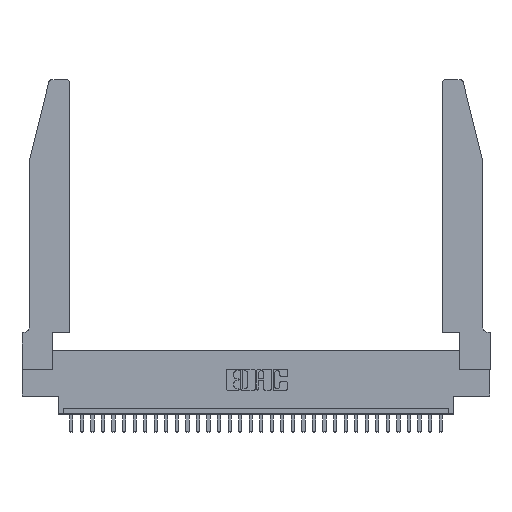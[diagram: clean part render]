
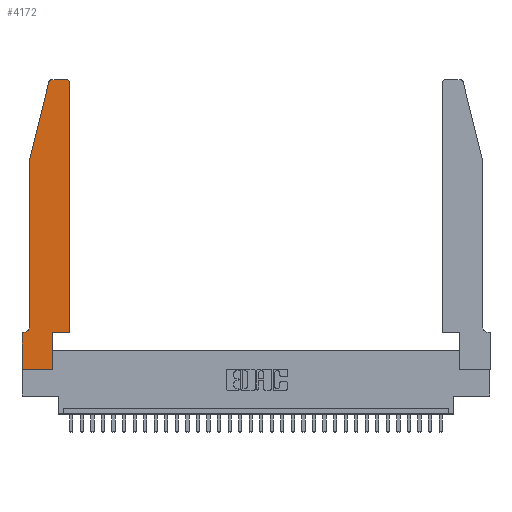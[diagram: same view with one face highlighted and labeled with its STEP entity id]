
A CAD part, top view. The second image highlights one B-rep face of the part: STEP entity #4172.
In plain terms, the highlighted planar face has unit normal (0, 0, 1).
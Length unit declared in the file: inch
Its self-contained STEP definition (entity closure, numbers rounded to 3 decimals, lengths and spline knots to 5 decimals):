
#710 = ORIENTED_EDGE ( 'NONE', *, *, #9412, .T. ) ;
#775 = AXIS2_PLACEMENT_3D ( 'NONE', #27414, #29863, #1965 ) ;
#939 = VECTOR ( 'NONE', #19447, 39.37008 ) ;
#1406 = CARTESIAN_POINT ( 'NONE',  ( 0.0755, 0.35, 0.37 ) ) ;
#1435 = ORIENTED_EDGE ( 'NONE', *, *, #9471, .T. ) ;
#1589 = DIRECTION ( 'NONE',  ( -0.239, -0.971, 0. ) ) ;
#1730 = VERTEX_POINT ( 'NONE', #30564 ) ;
#1965 = DIRECTION ( 'NONE',  ( -1., 0., 0. ) ) ;
#2129 = VERTEX_POINT ( 'NONE', #17123 ) ;
#2158 = CARTESIAN_POINT ( 'NONE',  ( 0.4505, 0.35, 0.37 ) ) ;
#2276 = EDGE_LOOP ( 'NONE', ( #29043, #710, #28399, #22956, #30868, #19934, #21627, #17759, #14311, #11859, #1435, #21307 ) ) ;
#2310 = CARTESIAN_POINT ( 'NONE',  ( 0., 0., 0.37 ) ) ;
#2598 = DIRECTION ( 'NONE',  ( 0., -1., 0. ) ) ;
#2951 = CARTESIAN_POINT ( 'NONE',  ( 0., 0., 0.37 ) ) ;
#3043 = DIRECTION ( 'NONE',  ( 0., -1., 0. ) ) ;
#3493 = VERTEX_POINT ( 'NONE', #13607 ) ;
#4172 = ADVANCED_FACE ( 'NONE', ( #28585 ), #24012, .T. ) ;
#4208 = DIRECTION ( 'NONE',  ( 0., 0., 1. ) ) ;
#4585 = AXIS2_PLACEMENT_3D ( 'NONE', #21987, #4208, #26896 ) ;
#4711 = LINE ( 'NONE', #12086, #24602 ) ;
#6222 = EDGE_CURVE ( 'NONE', #1730, #11894, #9465, .T. ) ;
#6285 = CARTESIAN_POINT ( 'NONE',  ( 0.0755, 2., 0.37 ) ) ;
#6349 = DIRECTION ( 'NONE',  ( 0., 0., 1. ) ) ;
#6385 = CARTESIAN_POINT ( 'NONE',  ( 0.4505, 2.72, 0.37 ) ) ;
#7360 = EDGE_CURVE ( 'NONE', #3493, #26805, #8144, .T. ) ;
#8144 = CIRCLE ( 'NONE', #775, 0.07 ) ;
#8229 = DIRECTION ( 'NONE',  ( -1., 0., 0. ) ) ;
#8315 = EDGE_CURVE ( 'NONE', #19337, #32767, #23153, .T. ) ;
#8439 = CARTESIAN_POINT ( 'NONE',  ( 0., 0., 0.37 ) ) ;
#8475 = LINE ( 'NONE', #2310, #20730 ) ;
#8700 = CARTESIAN_POINT ( 'NONE',  ( 0.284, 2.75, 0.37 ) ) ;
#9003 = VERTEX_POINT ( 'NONE', #6285 ) ;
#9332 = CARTESIAN_POINT ( 'NONE',  ( 0.2865, 0.35, 0.37 ) ) ;
#9412 = EDGE_CURVE ( 'NONE', #11894, #13403, #29058, .T. ) ;
#9465 = LINE ( 'NONE', #13617, #13462 ) ;
#9471 = EDGE_CURVE ( 'NONE', #18911, #9919, #30642, .T. ) ;
#9866 = CARTESIAN_POINT ( 'NONE',  ( 0.284, 2.72, 0.37 ) ) ;
#9919 = VERTEX_POINT ( 'NONE', #6385 ) ;
#9996 = DIRECTION ( 'NONE',  ( 1., 0., 0. ) ) ;
#10339 = EDGE_CURVE ( 'NONE', #13403, #9003, #4711, .T. ) ;
#11771 = LINE ( 'NONE', #2158, #13363 ) ;
#11859 = ORIENTED_EDGE ( 'NONE', *, *, #25365, .T. ) ;
#11894 = VERTEX_POINT ( 'NONE', #8700 ) ;
#12044 = LINE ( 'NONE', #25584, #17197 ) ;
#12086 = CARTESIAN_POINT ( 'NONE',  ( 0.0755, 2., 0.37 ) ) ;
#12638 = DIRECTION ( 'NONE',  ( 1., 0., 0. ) ) ;
#12874 = EDGE_CURVE ( 'NONE', #26805, #19337, #20810, .T. ) ;
#13363 = VECTOR ( 'NONE', #9996, 39.37008 ) ;
#13403 = VERTEX_POINT ( 'NONE', #19265 ) ;
#13462 = VECTOR ( 'NONE', #8229, 39.37008 ) ;
#13607 = CARTESIAN_POINT ( 'NONE',  ( 0.0755, 0.42, 0.37 ) ) ;
#13617 = CARTESIAN_POINT ( 'NONE',  ( 0.2605, 2.75, 0.37 ) ) ;
#13687 = VECTOR ( 'NONE', #3043, 39.37008 ) ;
#13959 = CARTESIAN_POINT ( 'NONE',  ( 0., 0.35, 0.37 ) ) ;
#14311 = ORIENTED_EDGE ( 'NONE', *, *, #24714, .T. ) ;
#17123 = CARTESIAN_POINT ( 'NONE',  ( 0.2865, 0., 0.37 ) ) ;
#17197 = VECTOR ( 'NONE', #2598, 39.37008 ) ;
#17759 = ORIENTED_EDGE ( 'NONE', *, *, #27505, .T. ) ;
#18055 = AXIS2_PLACEMENT_3D ( 'NONE', #9866, #22684, #12638 ) ;
#18151 = CARTESIAN_POINT ( 'NONE',  ( 0.4505, 0.35, 0.37 ) ) ;
#18911 = VERTEX_POINT ( 'NONE', #18151 ) ;
#19265 = CARTESIAN_POINT ( 'NONE',  ( 0.25487, 2.72718, 0.37 ) ) ;
#19278 = DIRECTION ( 'NONE',  ( 1., 0., 0. ) ) ;
#19337 = VERTEX_POINT ( 'NONE', #20521 ) ;
#19447 = DIRECTION ( 'NONE',  ( -1., 0., 0. ) ) ;
#19929 = VECTOR ( 'NONE', #27583, 39.37008 ) ;
#19934 = ORIENTED_EDGE ( 'NONE', *, *, #12874, .T. ) ;
#20521 = CARTESIAN_POINT ( 'NONE',  ( 0., 0.35, 0.37 ) ) ;
#20730 = VECTOR ( 'NONE', #25215, 39.37008 ) ;
#20810 = LINE ( 'NONE', #1406, #939 ) ;
#21307 = ORIENTED_EDGE ( 'NONE', *, *, #31254, .T. ) ;
#21627 = ORIENTED_EDGE ( 'NONE', *, *, #8315, .T. ) ;
#21987 = CARTESIAN_POINT ( 'NONE',  ( 0.4205, 2.72, 0.37 ) ) ;
#22684 = DIRECTION ( 'NONE',  ( 0., 0., 1. ) ) ;
#22956 = ORIENTED_EDGE ( 'NONE', *, *, #28137, .T. ) ;
#23153 = LINE ( 'NONE', #8439, #13687 ) ;
#23728 = VECTOR ( 'NONE', #23994, 39.37008 ) ;
#23893 = CARTESIAN_POINT ( 'NONE',  ( 0.2865, 0.35, 0.37 ) ) ;
#23994 = DIRECTION ( 'NONE',  ( 0., 1., 0. ) ) ;
#24012 = PLANE ( 'NONE',  #30506 ) ;
#24602 = VECTOR ( 'NONE', #1589, 39.37008 ) ;
#24714 = EDGE_CURVE ( 'NONE', #2129, #26265, #27276, .T. ) ;
#25215 = DIRECTION ( 'NONE',  ( 1., 0., 0. ) ) ;
#25273 = CIRCLE ( 'NONE', #4585, 0.03 ) ;
#25365 = EDGE_CURVE ( 'NONE', #26265, #18911, #11771, .T. ) ;
#25584 = CARTESIAN_POINT ( 'NONE',  ( 0.0755, 2., 0.37 ) ) ;
#26265 = VERTEX_POINT ( 'NONE', #9332 ) ;
#26805 = VERTEX_POINT ( 'NONE', #27907 ) ;
#26896 = DIRECTION ( 'NONE',  ( 1., 0., 0. ) ) ;
#27276 = LINE ( 'NONE', #23893, #23728 ) ;
#27414 = CARTESIAN_POINT ( 'NONE',  ( 0.0055, 0.42, 0.37 ) ) ;
#27505 = EDGE_CURVE ( 'NONE', #32767, #2129, #8475, .T. ) ;
#27583 = DIRECTION ( 'NONE',  ( 0., 1., 0. ) ) ;
#27907 = CARTESIAN_POINT ( 'NONE',  ( 0.0055, 0.35, 0.37 ) ) ;
#28137 = EDGE_CURVE ( 'NONE', #9003, #3493, #12044, .T. ) ;
#28399 = ORIENTED_EDGE ( 'NONE', *, *, #10339, .T. ) ;
#28585 = FACE_OUTER_BOUND ( 'NONE', #2276, .T. ) ;
#29043 = ORIENTED_EDGE ( 'NONE', *, *, #6222, .T. ) ;
#29058 = CIRCLE ( 'NONE', #18055, 0.03 ) ;
#29863 = DIRECTION ( 'NONE',  ( 0., 0., -1. ) ) ;
#30506 = AXIS2_PLACEMENT_3D ( 'NONE', #13959, #6349, #19278 ) ;
#30564 = CARTESIAN_POINT ( 'NONE',  ( 0.4205, 2.75, 0.37 ) ) ;
#30642 = LINE ( 'NONE', #32795, #19929 ) ;
#30868 = ORIENTED_EDGE ( 'NONE', *, *, #7360, .T. ) ;
#31254 = EDGE_CURVE ( 'NONE', #9919, #1730, #25273, .T. ) ;
#32767 = VERTEX_POINT ( 'NONE', #2951 ) ;
#32795 = CARTESIAN_POINT ( 'NONE',  ( 0.4505, 0.35, 0.37 ) ) ;
